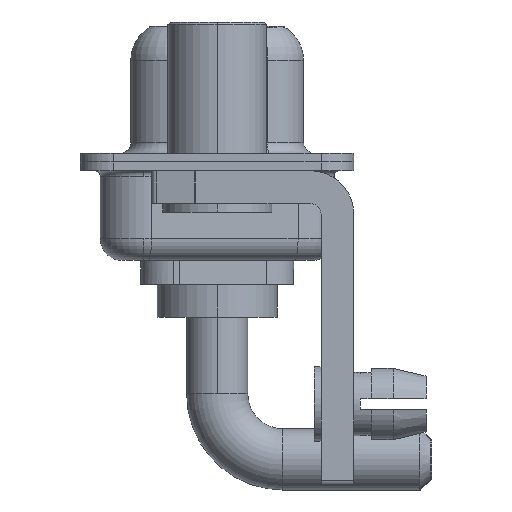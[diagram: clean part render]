
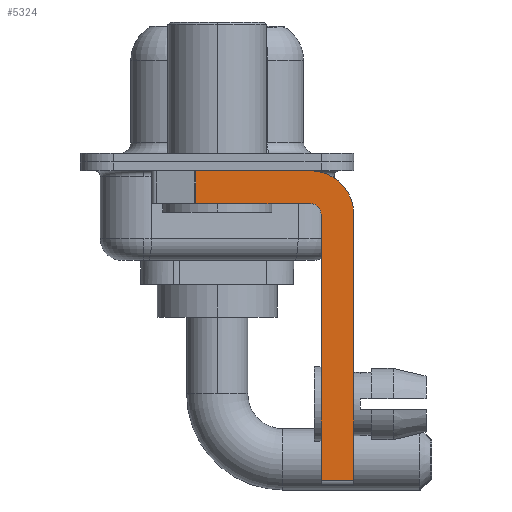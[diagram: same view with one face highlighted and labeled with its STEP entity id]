
A CAD part, left-side view. The second image highlights one B-rep face of the part: STEP entity #5324.
In plain terms, the highlighted planar face has unit normal (-1, 0, 0).
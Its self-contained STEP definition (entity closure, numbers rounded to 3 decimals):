
#6 = VECTOR ( 'NONE', #5776, 1000. ) ;
#172 = CARTESIAN_POINT ( 'NONE',  ( -2.9, -4.25, -0.4 ) ) ;
#349 = DIRECTION ( 'NONE',  ( 1., 0., 0. ) ) ;
#414 = EDGE_CURVE ( 'NONE', #16151, #10411, #8513, .T. ) ;
#462 = VECTOR ( 'NONE', #5657, 1000. ) ;
#1084 = ORIENTED_EDGE ( 'NONE', *, *, #9161, .F. ) ;
#1555 = AXIS2_PLACEMENT_3D ( 'NONE', #14455, #2777, #16071 ) ;
#1752 = ORIENTED_EDGE ( 'NONE', *, *, #2813, .T. ) ;
#2125 = VERTEX_POINT ( 'NONE', #7915 ) ;
#2235 = VECTOR ( 'NONE', #16488, 1000. ) ;
#2686 = CARTESIAN_POINT ( 'NONE',  ( -2.9, -6.25, -2.4 ) ) ;
#2777 = DIRECTION ( 'NONE',  ( -1., 0., 0. ) ) ;
#2813 = EDGE_CURVE ( 'NONE', #15478, #5563, #14102, .T. ) ;
#2973 = DIRECTION ( 'NONE',  ( 0., 0., -1. ) ) ;
#3348 = EDGE_CURVE ( 'NONE', #15478, #5257, #6093, .T. ) ;
#3629 = ORIENTED_EDGE ( 'NONE', *, *, #3876, .F. ) ;
#3876 = EDGE_CURVE ( 'NONE', #5040, #5563, #10566, .T. ) ;
#3900 = LINE ( 'NONE', #7752, #9339 ) ;
#4181 = EDGE_CURVE ( 'NONE', #16151, #2125, #3900, .T. ) ;
#4442 = CARTESIAN_POINT ( 'NONE',  ( -2.9, -6.25, -2.4 ) ) ;
#5040 = VERTEX_POINT ( 'NONE', #5904 ) ;
#5155 = DIRECTION ( 'NONE',  ( 0., 0., -1. ) ) ;
#5257 = VERTEX_POINT ( 'NONE', #172 ) ;
#5324 = ADVANCED_FACE ( 'NONE', ( #6744 ), #15799, .F. ) ;
#5474 = CIRCLE ( 'NONE', #13083, 2. ) ;
#5548 = VERTEX_POINT ( 'NONE', #4442 ) ;
#5563 = VERTEX_POINT ( 'NONE', #12861 ) ;
#5657 = DIRECTION ( 'NONE',  ( 0., 0., -1. ) ) ;
#5776 = DIRECTION ( 'NONE',  ( 0., 0., 1. ) ) ;
#5904 = CARTESIAN_POINT ( 'NONE',  ( -2.9, -4.25, -1.9 ) ) ;
#6093 = LINE ( 'NONE', #11283, #2235 ) ;
#6174 = CARTESIAN_POINT ( 'NONE',  ( -2.9, -4.75, -2.4 ) ) ;
#6334 = VECTOR ( 'NONE', #9300, 1000. ) ;
#6744 = FACE_OUTER_BOUND ( 'NONE', #10862, .T. ) ;
#7066 = EDGE_CURVE ( 'NONE', #5257, #5548, #5474, .T. ) ;
#7752 = CARTESIAN_POINT ( 'NONE',  ( -2.9, -4.25, -14.55 ) ) ;
#7910 = ORIENTED_EDGE ( 'NONE', *, *, #414, .F. ) ;
#7915 = CARTESIAN_POINT ( 'NONE',  ( -2.9, -6.25, -14.55 ) ) ;
#8048 = ORIENTED_EDGE ( 'NONE', *, *, #4181, .T. ) ;
#8147 = LINE ( 'NONE', #2686, #462 ) ;
#8188 = CARTESIAN_POINT ( 'NONE',  ( -2.9, -4.25, -1.9 ) ) ;
#8513 = LINE ( 'NONE', #9773, #6 ) ;
#9107 = EDGE_CURVE ( 'NONE', #5548, #2125, #8147, .T. ) ;
#9161 = EDGE_CURVE ( 'NONE', #10411, #5040, #11355, .T. ) ;
#9300 = DIRECTION ( 'NONE',  ( 0., 1., 0. ) ) ;
#9303 = DIRECTION ( 'NONE',  ( 1., 0., 0. ) ) ;
#9339 = VECTOR ( 'NONE', #15494, 1000. ) ;
#9481 = ORIENTED_EDGE ( 'NONE', *, *, #7066, .F. ) ;
#9773 = CARTESIAN_POINT ( 'NONE',  ( -2.9, -4.75, -14.8 ) ) ;
#10109 = VECTOR ( 'NONE', #5155, 1000. ) ;
#10411 = VERTEX_POINT ( 'NONE', #6174 ) ;
#10480 = CARTESIAN_POINT ( 'NONE',  ( -2.9, -4.75, -14.55 ) ) ;
#10566 = LINE ( 'NONE', #8188, #6334 ) ;
#10862 = EDGE_LOOP ( 'NONE', ( #12746, #1752, #3629, #1084, #7910, #8048, #14503, #9481 ) ) ;
#11283 = CARTESIAN_POINT ( 'NONE',  ( -2.9, 3., -0.4 ) ) ;
#11355 = CIRCLE ( 'NONE', #1555, 0.5 ) ;
#11426 = AXIS2_PLACEMENT_3D ( 'NONE', #12029, #349, #14672 ) ;
#12029 = CARTESIAN_POINT ( 'NONE',  ( -2.9, -4.25, -2.4 ) ) ;
#12746 = ORIENTED_EDGE ( 'NONE', *, *, #3348, .F. ) ;
#12861 = CARTESIAN_POINT ( 'NONE',  ( -2.9, 0.978, -1.9 ) ) ;
#13083 = AXIS2_PLACEMENT_3D ( 'NONE', #14655, #9303, #2973 ) ;
#14102 = LINE ( 'NONE', #16827, #10109 ) ;
#14455 = CARTESIAN_POINT ( 'NONE',  ( -2.9, -4.25, -2.4 ) ) ;
#14503 = ORIENTED_EDGE ( 'NONE', *, *, #9107, .F. ) ;
#14655 = CARTESIAN_POINT ( 'NONE',  ( -2.9, -4.25, -2.4 ) ) ;
#14672 = DIRECTION ( 'NONE',  ( 0., 0., -1. ) ) ;
#15370 = CARTESIAN_POINT ( 'NONE',  ( -2.9, 0.978, -0.4 ) ) ;
#15478 = VERTEX_POINT ( 'NONE', #15370 ) ;
#15494 = DIRECTION ( 'NONE',  ( 0., -1., 0. ) ) ;
#15799 = PLANE ( 'NONE',  #11426 ) ;
#16071 = DIRECTION ( 'NONE',  ( 0., 0., 1. ) ) ;
#16151 = VERTEX_POINT ( 'NONE', #10480 ) ;
#16488 = DIRECTION ( 'NONE',  ( 0., -1., 0. ) ) ;
#16827 = CARTESIAN_POINT ( 'NONE',  ( -2.9, 0.978, -1.9 ) ) ;
